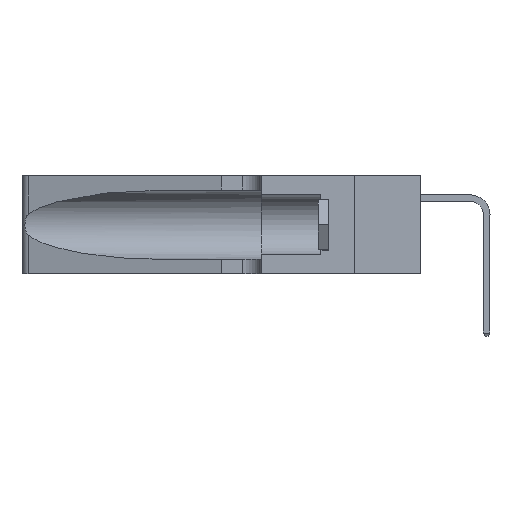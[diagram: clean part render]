
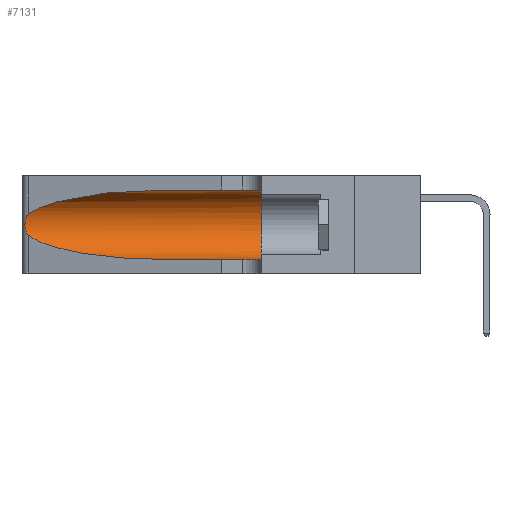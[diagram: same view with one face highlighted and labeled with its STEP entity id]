
A CAD part, left-side view. The second image highlights one B-rep face of the part: STEP entity #7131.
In plain terms, the highlighted cylindrical face has radius 3.308 mm (diameter 6.617 mm), a partial arc.
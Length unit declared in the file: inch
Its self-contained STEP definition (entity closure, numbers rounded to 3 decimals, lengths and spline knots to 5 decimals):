
#174 = LINE ( 'NONE', #3150, #16800 ) ;
#557 = CIRCLE ( 'NONE', #4340, 0.13025 ) ;
#1076 = CARTESIAN_POINT ( 'NONE',  ( 0.2373, 1.15595, 0.28018 ) ) ;
#1370 = CARTESIAN_POINT ( 'NONE',  ( 0.25555, 1.22993, 0.14849 ) ) ;
#2102 = VERTEX_POINT ( 'NONE', #13011 ) ;
#2488 = VERTEX_POINT ( 'NONE', #20734 ) ;
#2578 = EDGE_CURVE ( 'NONE', #2851, #19486, #14073, .T. ) ;
#2851 = VERTEX_POINT ( 'NONE', #8515 ) ;
#2989 = CARTESIAN_POINT ( 'NONE',  ( 0.25555, 1.22994, 0.2215 ) ) ;
#3150 = CARTESIAN_POINT ( 'NONE',  ( 0.1305, 1.61858, 0.31525 ) ) ;
#3238 = DIRECTION ( 'NONE',  ( 0., 0., -1. ) ) ;
#3382 = FACE_OUTER_BOUND ( 'NONE', #18645, .T. ) ;
#3864 = CARTESIAN_POINT ( 'NONE',  ( 0.1305, 0.35, 0.185 ) ) ;
#4340 = AXIS2_PLACEMENT_3D ( 'NONE', #3864, #15453, #5550 ) ;
#4506 = ORIENTED_EDGE ( 'NONE', *, *, #19928, .T. ) ;
#4683 = CARTESIAN_POINT ( 'NONE',  ( 0.25787, 1.23484, 0.2124 ) ) ;
#4934 = DIRECTION ( 'NONE',  ( 0., -1., 0. ) ) ;
#5112 = EDGE_CURVE ( 'NONE', #2488, #2102, #557, .T. ) ;
#5217 = CARTESIAN_POINT ( 'NONE',  ( 0.2373, 1.15595, 0.08982 ) ) ;
#5550 = DIRECTION ( 'NONE',  ( 0., 0., 1. ) ) ;
#5744 =( BOUNDED_CURVE ( )  B_SPLINE_CURVE ( 3, ( #13437, #5217, #16775, #6877 ),
 .UNSPECIFIED., .F., .F. ) 
 B_SPLINE_CURVE_WITH_KNOTS ( ( 4, 4 ),
 ( 3.44316, 4.71239 ),
 .UNSPECIFIED. ) 
 CURVE ( )  GEOMETRIC_REPRESENTATION_ITEM ( )  RATIONAL_B_SPLINE_CURVE ( ( 1., 0.87, 0.87, 1. ) ) 
 REPRESENTATION_ITEM ( '' )  );
#6356 = CARTESIAN_POINT ( 'NONE',  ( 0.26018, 1.23835, 0.19895 ) ) ;
#6829 = ORIENTED_EDGE ( 'NONE', *, *, #2578, .T. ) ;
#6877 = CARTESIAN_POINT ( 'NONE',  ( 0.1305, 0.72297, 0.05475 ) ) ;
#7131 = ADVANCED_FACE ( 'NONE', ( #3382 ), #16087, .F. ) ;
#7998 = CARTESIAN_POINT ( 'NONE',  ( 0.26075, 1.23896, 0.178 ) ) ;
#8515 = CARTESIAN_POINT ( 'NONE',  ( 0.1305, 0.72297, 0.31525 ) ) ;
#8592 = VERTEX_POINT ( 'NONE', #20134 ) ;
#8812 = AXIS2_PLACEMENT_3D ( 'NONE', #11506, #4934, #3238 ) ;
#9656 = CARTESIAN_POINT ( 'NONE',  ( 0.25856, 1.23593, 0.16098 ) ) ;
#11242 = CARTESIAN_POINT ( 'NONE',  ( 0.25487, 1.22718, 0.22369 ) ) ;
#11314 = CARTESIAN_POINT ( 'NONE',  ( 0.25639, 1.23186, 0.15144 ) ) ;
#11497 = ORIENTED_EDGE ( 'NONE', *, *, #19529, .T. ) ;
#11506 = CARTESIAN_POINT ( 'NONE',  ( 0.1305, 1.61858, 0.185 ) ) ;
#12421 = CARTESIAN_POINT ( 'NONE',  ( 0.1305, 1.61858, 0.05475 ) ) ;
#12695 = CARTESIAN_POINT ( 'NONE',  ( 0.1305, 0.72297, 0.31525 ) ) ;
#12979 = CARTESIAN_POINT ( 'NONE',  ( 0.25487, 1.22718, 0.14631 ) ) ;
#13011 = CARTESIAN_POINT ( 'NONE',  ( 0.1305, 0.35, 0.05475 ) ) ;
#13050 = ORIENTED_EDGE ( 'NONE', *, *, #17025, .F. ) ;
#13085 = DIRECTION ( 'NONE',  ( 0., -1., 0. ) ) ;
#13437 = CARTESIAN_POINT ( 'NONE',  ( 0.25487, 1.22718, 0.14631 ) ) ;
#14073 =( BOUNDED_CURVE ( )  B_SPLINE_CURVE ( 3, ( #12695, #20957, #1076, #14363 ),
 .UNSPECIFIED., .F., .F. ) 
 B_SPLINE_CURVE_WITH_KNOTS ( ( 4, 4 ),
 ( 1.5708, 2.84003 ),
 .UNSPECIFIED. ) 
 CURVE ( )  GEOMETRIC_REPRESENTATION_ITEM ( )  RATIONAL_B_SPLINE_CURVE ( ( 1., 0.87, 0.87, 1. ) ) 
 REPRESENTATION_ITEM ( '' )  );
#14363 = CARTESIAN_POINT ( 'NONE',  ( 0.25487, 1.22718, 0.22369 ) ) ;
#14557 = CARTESIAN_POINT ( 'NONE',  ( 0.25639, 1.23184, 0.21858 ) ) ;
#15391 = VERTEX_POINT ( 'NONE', #18952 ) ;
#15453 = DIRECTION ( 'NONE',  ( 0., 1., 0. ) ) ;
#15633 = CARTESIAN_POINT ( 'NONE',  ( 0.25487, 1.22718, 0.22369 ) ) ;
#15682 = B_SPLINE_CURVE_WITH_KNOTS ( 'NONE', 3,
 ( #11242, #2989, #14557, #4683, #16250, #6356, #17898, #7998, #19576, #9656, #21238, #11314, #1370, #12979 ),
 .UNSPECIFIED., .F., .F.,
 ( 4, 2, 2, 2, 2, 2, 4 ),
 ( 0., 0.00027, 0.00053, 0.00107, 0.0016, 0.00187, 0.00214 ),
 .UNSPECIFIED. ) ;
#15794 = EDGE_CURVE ( 'NONE', #19486, #8592, #15682, .T. ) ;
#16087 = CYLINDRICAL_SURFACE ( 'NONE', #8812, 0.13025 ) ;
#16250 = CARTESIAN_POINT ( 'NONE',  ( 0.25854, 1.2359, 0.20912 ) ) ;
#16775 = CARTESIAN_POINT ( 'NONE',  ( 0.18966, 0.96281, 0.05475 ) ) ;
#16800 = VECTOR ( 'NONE', #13085, 39.37008 ) ;
#17025 = EDGE_CURVE ( 'NONE', #2851, #2488, #174, .T. ) ;
#17438 = DIRECTION ( 'NONE',  ( 0., -1., 0. ) ) ;
#17898 = CARTESIAN_POINT ( 'NONE',  ( 0.26075, 1.23896, 0.19203 ) ) ;
#18229 = VECTOR ( 'NONE', #17438, 39.37008 ) ;
#18645 = EDGE_LOOP ( 'NONE', ( #6829, #21045, #4506, #11497, #20814, #13050 ) ) ;
#18762 = LINE ( 'NONE', #12421, #18229 ) ;
#18952 = CARTESIAN_POINT ( 'NONE',  ( 0.1305, 0.72297, 0.05475 ) ) ;
#19486 = VERTEX_POINT ( 'NONE', #15633 ) ;
#19529 = EDGE_CURVE ( 'NONE', #15391, #2102, #18762, .T. ) ;
#19576 = CARTESIAN_POINT ( 'NONE',  ( 0.26017, 1.23833, 0.17102 ) ) ;
#19928 = EDGE_CURVE ( 'NONE', #8592, #15391, #5744, .T. ) ;
#20134 = CARTESIAN_POINT ( 'NONE',  ( 0.25487, 1.22718, 0.14631 ) ) ;
#20734 = CARTESIAN_POINT ( 'NONE',  ( 0.1305, 0.35, 0.31525 ) ) ;
#20814 = ORIENTED_EDGE ( 'NONE', *, *, #5112, .F. ) ;
#20957 = CARTESIAN_POINT ( 'NONE',  ( 0.18966, 0.96281, 0.31525 ) ) ;
#21045 = ORIENTED_EDGE ( 'NONE', *, *, #15794, .T. ) ;
#21238 = CARTESIAN_POINT ( 'NONE',  ( 0.25789, 1.23486, 0.15765 ) ) ;
